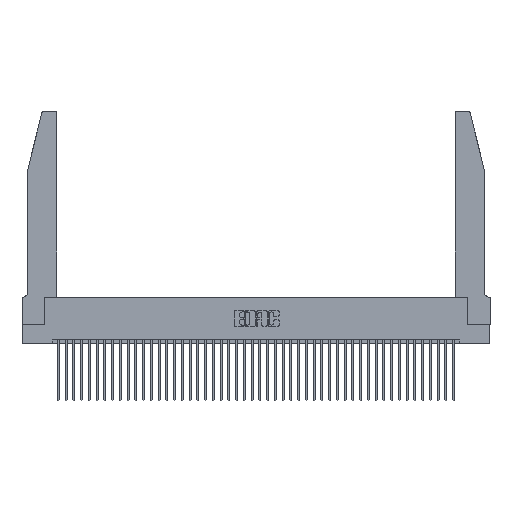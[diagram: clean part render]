
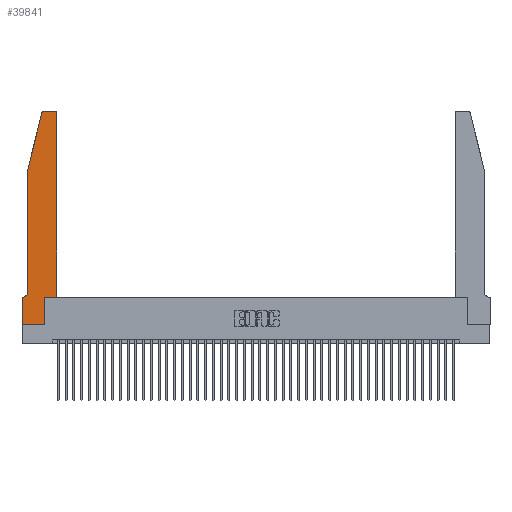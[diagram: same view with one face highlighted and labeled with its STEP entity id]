
A CAD part, top view. The second image highlights one B-rep face of the part: STEP entity #39841.
In plain terms, the highlighted planar face has unit normal (0, 0, 1).
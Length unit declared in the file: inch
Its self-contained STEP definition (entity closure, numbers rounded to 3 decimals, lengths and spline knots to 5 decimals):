
#52 = DIRECTION ( 'NONE',  ( -0.239, -0.971, 0. ) ) ;
#324 = EDGE_LOOP ( 'NONE', ( #7396, #25711, #27790, #1484, #3648, #22024, #30940, #25209, #43193, #29375, #3142, #30441 ) ) ;
#707 = DIRECTION ( 'NONE',  ( -1., 0., 0. ) ) ;
#755 = CARTESIAN_POINT ( 'NONE',  ( 0.0755, 2., 0.37 ) ) ;
#1484 = ORIENTED_EDGE ( 'NONE', *, *, #4301, .T. ) ;
#1661 = LINE ( 'NONE', #25802, #10812 ) ;
#3142 = ORIENTED_EDGE ( 'NONE', *, *, #41012, .T. ) ;
#3381 = DIRECTION ( 'NONE',  ( 0., 1., 0. ) ) ;
#3396 = FACE_OUTER_BOUND ( 'NONE', #324, .T. ) ;
#3648 = ORIENTED_EDGE ( 'NONE', *, *, #9623, .T. ) ;
#4301 = EDGE_CURVE ( 'NONE', #13853, #13630, #16562, .T. ) ;
#4362 = EDGE_CURVE ( 'NONE', #8272, #10969, #6243, .T. ) ;
#4965 = VERTEX_POINT ( 'NONE', #29169 ) ;
#5176 = CARTESIAN_POINT ( 'NONE',  ( 0.0055, 0.42, 0.37 ) ) ;
#5669 = VERTEX_POINT ( 'NONE', #19237 ) ;
#6243 = LINE ( 'NONE', #18411, #14335 ) ;
#7396 = ORIENTED_EDGE ( 'NONE', *, *, #21779, .T. ) ;
#7973 = CIRCLE ( 'NONE', #28966, 0.07 ) ;
#8272 = VERTEX_POINT ( 'NONE', #34070 ) ;
#8295 = LINE ( 'NONE', #27698, #33432 ) ;
#8361 = CARTESIAN_POINT ( 'NONE',  ( 0., 0., 0.37 ) ) ;
#8598 = CIRCLE ( 'NONE', #39448, 0.03 ) ;
#8633 = DIRECTION ( 'NONE',  ( -1., 0., 0. ) ) ;
#8882 = EDGE_CURVE ( 'NONE', #5669, #8272, #18908, .T. ) ;
#9623 = EDGE_CURVE ( 'NONE', #13630, #22588, #7973, .T. ) ;
#9630 = DIRECTION ( 'NONE',  ( 0., 0., 1. ) ) ;
#10604 = DIRECTION ( 'NONE',  ( 0., -1., 0. ) ) ;
#10812 = VECTOR ( 'NONE', #29143, 39.37008 ) ;
#10969 = VERTEX_POINT ( 'NONE', #22604 ) ;
#11944 = VERTEX_POINT ( 'NONE', #34611 ) ;
#12547 = LINE ( 'NONE', #24154, #31736 ) ;
#12811 = CARTESIAN_POINT ( 'NONE',  ( 0.284, 2.75, 0.37 ) ) ;
#13352 = CARTESIAN_POINT ( 'NONE',  ( 0.4205, 2.72, 0.37 ) ) ;
#13630 = VERTEX_POINT ( 'NONE', #41123 ) ;
#13853 = VERTEX_POINT ( 'NONE', #28923 ) ;
#13948 = EDGE_CURVE ( 'NONE', #22588, #29691, #40675, .T. ) ;
#14335 = VECTOR ( 'NONE', #25128, 39.37008 ) ;
#15440 = VECTOR ( 'NONE', #35018, 39.37008 ) ;
#15918 = CARTESIAN_POINT ( 'NONE',  ( 0., 0.35, 0.37 ) ) ;
#15934 = VECTOR ( 'NONE', #38699, 39.37008 ) ;
#16562 = LINE ( 'NONE', #755, #15440 ) ;
#16642 = EDGE_CURVE ( 'NONE', #30649, #4965, #23175, .T. ) ;
#16858 = DIRECTION ( 'NONE',  ( 1., 0., 0. ) ) ;
#17319 = CARTESIAN_POINT ( 'NONE',  ( 0.4505, 2.72, 0.37 ) ) ;
#18044 = VERTEX_POINT ( 'NONE', #8361 ) ;
#18411 = CARTESIAN_POINT ( 'NONE',  ( 0.4505, 0.35, 0.37 ) ) ;
#18908 = LINE ( 'NONE', #20781, #38009 ) ;
#19237 = CARTESIAN_POINT ( 'NONE',  ( 0.2865, 0., 0.37 ) ) ;
#19333 = DIRECTION ( 'NONE',  ( -1., 0., 0. ) ) ;
#19549 = CARTESIAN_POINT ( 'NONE',  ( 0.284, 2.72, 0.37 ) ) ;
#20781 = CARTESIAN_POINT ( 'NONE',  ( 0.2865, 0.35, 0.37 ) ) ;
#21158 = EDGE_CURVE ( 'NONE', #11944, #13853, #12547, .T. ) ;
#21410 = CARTESIAN_POINT ( 'NONE',  ( 0.2605, 2.75, 0.37 ) ) ;
#21779 = EDGE_CURVE ( 'NONE', #4965, #22763, #24373, .T. ) ;
#22024 = ORIENTED_EDGE ( 'NONE', *, *, #13948, .T. ) ;
#22588 = VERTEX_POINT ( 'NONE', #35650 ) ;
#22604 = CARTESIAN_POINT ( 'NONE',  ( 0.4505, 0.35, 0.37 ) ) ;
#22763 = VERTEX_POINT ( 'NONE', #12811 ) ;
#22986 = DIRECTION ( 'NONE',  ( 1., 0., 0. ) ) ;
#23175 = CIRCLE ( 'NONE', #30249, 0.03 ) ;
#24154 = CARTESIAN_POINT ( 'NONE',  ( 0.0755, 2., 0.37 ) ) ;
#24373 = LINE ( 'NONE', #21410, #41287 ) ;
#25063 = LINE ( 'NONE', #31818, #15934 ) ;
#25128 = DIRECTION ( 'NONE',  ( 1., 0., 0. ) ) ;
#25209 = ORIENTED_EDGE ( 'NONE', *, *, #27069, .T. ) ;
#25711 = ORIENTED_EDGE ( 'NONE', *, *, #31091, .T. ) ;
#25802 = CARTESIAN_POINT ( 'NONE',  ( 0.4505, 0.35, 0.37 ) ) ;
#26762 = PLANE ( 'NONE',  #30538 ) ;
#27069 = EDGE_CURVE ( 'NONE', #18044, #5669, #25063, .T. ) ;
#27698 = CARTESIAN_POINT ( 'NONE',  ( 0., 0., 0.37 ) ) ;
#27790 = ORIENTED_EDGE ( 'NONE', *, *, #21158, .T. ) ;
#28923 = CARTESIAN_POINT ( 'NONE',  ( 0.0755, 2., 0.37 ) ) ;
#28966 = AXIS2_PLACEMENT_3D ( 'NONE', #5176, #29146, #8633 ) ;
#29143 = DIRECTION ( 'NONE',  ( 0., 1., 0. ) ) ;
#29146 = DIRECTION ( 'NONE',  ( 0., 0., -1. ) ) ;
#29169 = CARTESIAN_POINT ( 'NONE',  ( 0.4205, 2.75, 0.37 ) ) ;
#29375 = ORIENTED_EDGE ( 'NONE', *, *, #4362, .T. ) ;
#29691 = VERTEX_POINT ( 'NONE', #15918 ) ;
#30249 = AXIS2_PLACEMENT_3D ( 'NONE', #13352, #37214, #16858 ) ;
#30441 = ORIENTED_EDGE ( 'NONE', *, *, #16642, .T. ) ;
#30538 = AXIS2_PLACEMENT_3D ( 'NONE', #36831, #9630, #33530 ) ;
#30649 = VERTEX_POINT ( 'NONE', #17319 ) ;
#30940 = ORIENTED_EDGE ( 'NONE', *, *, #34349, .T. ) ;
#31091 = EDGE_CURVE ( 'NONE', #22763, #11944, #8598, .T. ) ;
#31576 = VECTOR ( 'NONE', #19333, 39.37008 ) ;
#31736 = VECTOR ( 'NONE', #52, 39.37008 ) ;
#31818 = CARTESIAN_POINT ( 'NONE',  ( 0., 0., 0.37 ) ) ;
#33432 = VECTOR ( 'NONE', #10604, 39.37008 ) ;
#33530 = DIRECTION ( 'NONE',  ( 1., 0., 0. ) ) ;
#34070 = CARTESIAN_POINT ( 'NONE',  ( 0.2865, 0.35, 0.37 ) ) ;
#34349 = EDGE_CURVE ( 'NONE', #29691, #18044, #8295, .T. ) ;
#34611 = CARTESIAN_POINT ( 'NONE',  ( 0.25487, 2.72718, 0.37 ) ) ;
#35018 = DIRECTION ( 'NONE',  ( 0., -1., 0. ) ) ;
#35650 = CARTESIAN_POINT ( 'NONE',  ( 0.0055, 0.35, 0.37 ) ) ;
#36831 = CARTESIAN_POINT ( 'NONE',  ( 0., 0.35, 0.37 ) ) ;
#37214 = DIRECTION ( 'NONE',  ( 0., 0., 1. ) ) ;
#38009 = VECTOR ( 'NONE', #3381, 39.37008 ) ;
#38699 = DIRECTION ( 'NONE',  ( 1., 0., 0. ) ) ;
#39448 = AXIS2_PLACEMENT_3D ( 'NONE', #19549, #43225, #22986 ) ;
#39628 = CARTESIAN_POINT ( 'NONE',  ( 0.0755, 0.35, 0.37 ) ) ;
#39841 = ADVANCED_FACE ( 'NONE', ( #3396 ), #26762, .T. ) ;
#40675 = LINE ( 'NONE', #39628, #31576 ) ;
#41012 = EDGE_CURVE ( 'NONE', #10969, #30649, #1661, .T. ) ;
#41123 = CARTESIAN_POINT ( 'NONE',  ( 0.0755, 0.42, 0.37 ) ) ;
#41287 = VECTOR ( 'NONE', #707, 39.37008 ) ;
#43193 = ORIENTED_EDGE ( 'NONE', *, *, #8882, .T. ) ;
#43225 = DIRECTION ( 'NONE',  ( 0., 0., 1. ) ) ;
